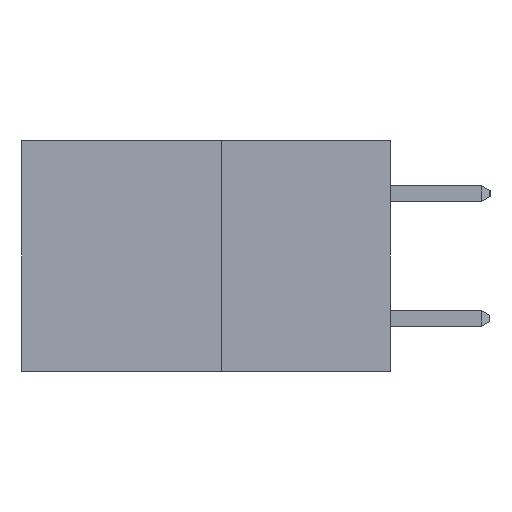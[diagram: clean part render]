
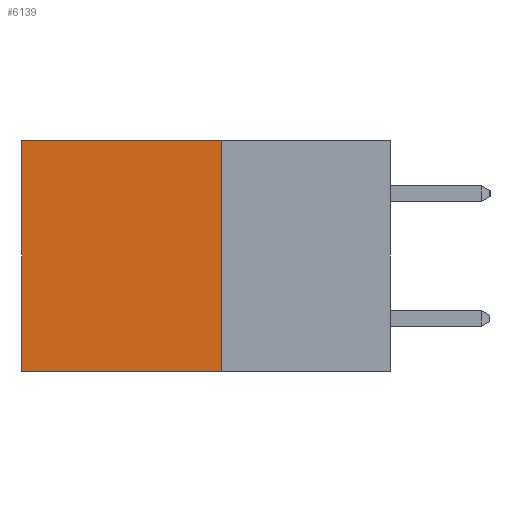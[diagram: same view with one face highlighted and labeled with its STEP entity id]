
A CAD part, left-side view. The second image highlights one B-rep face of the part: STEP entity #6139.
In plain terms, the highlighted planar face has unit normal (-1, 0, 0).
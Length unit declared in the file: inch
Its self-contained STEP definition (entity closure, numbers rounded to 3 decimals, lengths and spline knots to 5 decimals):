
#241 = VECTOR ( 'NONE', #13974, 39.37008 ) ;
#652 = EDGE_CURVE ( 'NONE', #15058, #14047, #4101, .T. ) ;
#1227 = ORIENTED_EDGE ( 'NONE', *, *, #8468, .F. ) ;
#1696 = CARTESIAN_POINT ( 'NONE',  ( 0.277, 0.59, -0.37 ) ) ;
#2676 = DIRECTION ( 'NONE',  ( 0., 0., -1. ) ) ;
#2819 = CARTESIAN_POINT ( 'NONE',  ( 0.277, 0.27, 0. ) ) ;
#3372 = FACE_OUTER_BOUND ( 'NONE', #9730, .T. ) ;
#3478 = LINE ( 'NONE', #1696, #241 ) ;
#3641 = CARTESIAN_POINT ( 'NONE',  ( 0.277, 0.27, 0. ) ) ;
#3731 = ORIENTED_EDGE ( 'NONE', *, *, #12530, .T. ) ;
#4101 = LINE ( 'NONE', #3641, #10665 ) ;
#5529 = DIRECTION ( 'NONE',  ( 0., 0., -1. ) ) ;
#6139 = ADVANCED_FACE ( 'NONE', ( #3372 ), #8811, .F. ) ;
#6366 = CARTESIAN_POINT ( 'NONE',  ( 0.277, 0.27, -0.37 ) ) ;
#6606 = DIRECTION ( 'NONE',  ( 0., 1., 0. ) ) ;
#7096 = AXIS2_PLACEMENT_3D ( 'NONE', #14797, #10036, #2676 ) ;
#7102 = CARTESIAN_POINT ( 'NONE',  ( 0.277, 0.59, 0. ) ) ;
#7557 = VECTOR ( 'NONE', #6606, 39.37008 ) ;
#8468 = EDGE_CURVE ( 'NONE', #15058, #13632, #14702, .T. ) ;
#8781 = VERTEX_POINT ( 'NONE', #11243 ) ;
#8811 = PLANE ( 'NONE',  #7096 ) ;
#9730 = EDGE_LOOP ( 'NONE', ( #3731, #9893, #1227, #14804 ) ) ;
#9893 = ORIENTED_EDGE ( 'NONE', *, *, #12035, .F. ) ;
#10036 = DIRECTION ( 'NONE',  ( 1., 0., 0. ) ) ;
#10303 = CARTESIAN_POINT ( 'NONE',  ( 0.277, 0.27, -0.37 ) ) ;
#10435 = LINE ( 'NONE', #10303, #7557 ) ;
#10665 = VECTOR ( 'NONE', #14416, 39.37008 ) ;
#11243 = CARTESIAN_POINT ( 'NONE',  ( 0.277, 0.59, -0.37 ) ) ;
#11496 = VECTOR ( 'NONE', #5529, 39.37008 ) ;
#11922 = CARTESIAN_POINT ( 'NONE',  ( 0.277, 0.27, -0.37 ) ) ;
#12035 = EDGE_CURVE ( 'NONE', #13632, #8781, #10435, .T. ) ;
#12530 = EDGE_CURVE ( 'NONE', #14047, #8781, #3478, .T. ) ;
#13632 = VERTEX_POINT ( 'NONE', #6366 ) ;
#13974 = DIRECTION ( 'NONE',  ( 0., 0., -1. ) ) ;
#14047 = VERTEX_POINT ( 'NONE', #7102 ) ;
#14416 = DIRECTION ( 'NONE',  ( 0., 1., 0. ) ) ;
#14702 = LINE ( 'NONE', #11922, #11496 ) ;
#14797 = CARTESIAN_POINT ( 'NONE',  ( 0.277, 0.27, -0.37 ) ) ;
#14804 = ORIENTED_EDGE ( 'NONE', *, *, #652, .T. ) ;
#15058 = VERTEX_POINT ( 'NONE', #2819 ) ;
